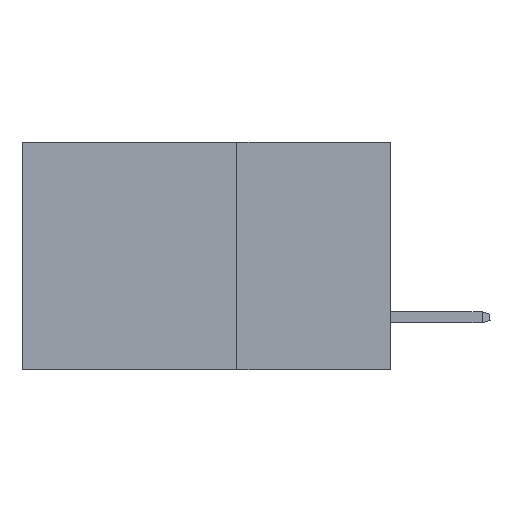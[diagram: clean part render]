
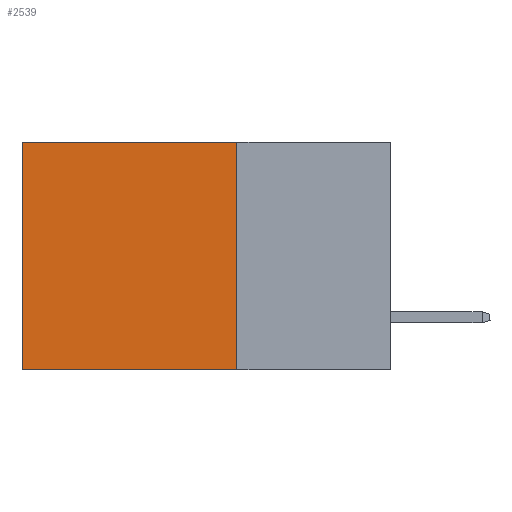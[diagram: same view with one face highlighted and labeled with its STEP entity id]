
A CAD part, left-side view. The second image highlights one B-rep face of the part: STEP entity #2539.
In plain terms, the highlighted planar face has unit normal (-1, 0, 0).
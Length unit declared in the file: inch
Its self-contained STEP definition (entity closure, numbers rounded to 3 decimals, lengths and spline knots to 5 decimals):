
#1 = DIRECTION ( 'NONE',  ( 0., 1., 0. ) ) ;
#56 = VERTEX_POINT ( 'NONE', #12697 ) ;
#305 = ORIENTED_EDGE ( 'NONE', *, *, #2394, .F. ) ;
#335 = LINE ( 'NONE', #22023, #3960 ) ;
#609 = AXIS2_PLACEMENT_3D ( 'NONE', #20880, #1804, #3765 ) ;
#1704 = ORIENTED_EDGE ( 'NONE', *, *, #15354, .T. ) ;
#1804 = DIRECTION ( 'NONE',  ( 1., 0., 0. ) ) ;
#2394 = EDGE_CURVE ( 'NONE', #6447, #23059, #8750, .T. ) ;
#2539 = ADVANCED_FACE ( 'NONE', ( #23182 ), #13325, .F. ) ;
#2822 = CARTESIAN_POINT ( 'NONE',  ( 0.2875, 0.25, 0. ) ) ;
#3672 = EDGE_CURVE ( 'NONE', #6594, #56, #24894, .T. ) ;
#3765 = DIRECTION ( 'NONE',  ( 0., 0., -1. ) ) ;
#3960 = VECTOR ( 'NONE', #10355, 39.37008 ) ;
#5353 = CARTESIAN_POINT ( 'NONE',  ( 0.2875, 0.25, -0.37 ) ) ;
#6447 = VERTEX_POINT ( 'NONE', #11507 ) ;
#6594 = VERTEX_POINT ( 'NONE', #2822 ) ;
#7438 = CARTESIAN_POINT ( 'NONE',  ( 0.2875, 0.25, 0. ) ) ;
#8750 = LINE ( 'NONE', #5353, #23456 ) ;
#10355 = DIRECTION ( 'NONE',  ( 0., 0., -1. ) ) ;
#11507 = CARTESIAN_POINT ( 'NONE',  ( 0.2875, 0.25, -0.37 ) ) ;
#11698 = VECTOR ( 'NONE', #1, 39.37008 ) ;
#12697 = CARTESIAN_POINT ( 'NONE',  ( 0.2875, 0.6, 0. ) ) ;
#13325 = PLANE ( 'NONE',  #609 ) ;
#13632 = CARTESIAN_POINT ( 'NONE',  ( 0.2875, 0.25, 0. ) ) ;
#13842 = ORIENTED_EDGE ( 'NONE', *, *, #24405, .F. ) ;
#14593 = ORIENTED_EDGE ( 'NONE', *, *, #3672, .T. ) ;
#14849 = DIRECTION ( 'NONE',  ( 0., 1., 0. ) ) ;
#15354 = EDGE_CURVE ( 'NONE', #56, #23059, #335, .T. ) ;
#20038 = LINE ( 'NONE', #7438, #20639 ) ;
#20519 = DIRECTION ( 'NONE',  ( 0., 0., -1. ) ) ;
#20627 = EDGE_LOOP ( 'NONE', ( #1704, #305, #13842, #14593 ) ) ;
#20639 = VECTOR ( 'NONE', #20519, 39.37008 ) ;
#20880 = CARTESIAN_POINT ( 'NONE',  ( 0.2875, 0.25, 0. ) ) ;
#21212 = CARTESIAN_POINT ( 'NONE',  ( 0.2875, 0.6, -0.37 ) ) ;
#22023 = CARTESIAN_POINT ( 'NONE',  ( 0.2875, 0.6, 0. ) ) ;
#23059 = VERTEX_POINT ( 'NONE', #21212 ) ;
#23182 = FACE_OUTER_BOUND ( 'NONE', #20627, .T. ) ;
#23456 = VECTOR ( 'NONE', #14849, 39.37008 ) ;
#24405 = EDGE_CURVE ( 'NONE', #6594, #6447, #20038, .T. ) ;
#24894 = LINE ( 'NONE', #13632, #11698 ) ;
